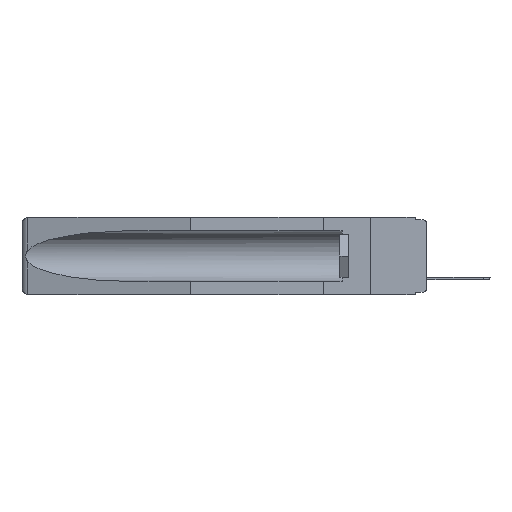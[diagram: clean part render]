
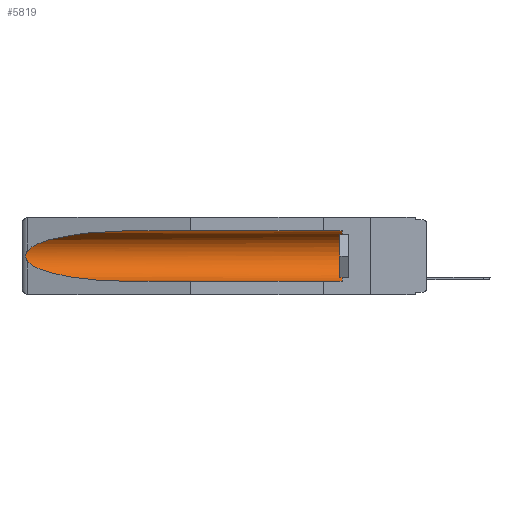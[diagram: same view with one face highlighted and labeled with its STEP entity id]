
A CAD part, left-side view. The second image highlights one B-rep face of the part: STEP entity #5819.
In plain terms, the highlighted cylindrical face has radius 2.857 mm (diameter 5.715 mm), a partial arc.
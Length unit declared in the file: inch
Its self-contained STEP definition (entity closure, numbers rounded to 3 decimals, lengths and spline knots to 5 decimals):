
#19 = CARTESIAN_POINT ( 'NONE',  ( 0.26537, 1.52718, -0.19328 ) ) ;
#330 = CARTESIAN_POINT ( 'NONE',  ( 0.26537, 1.52718, -0.14972 ) ) ;
#913 = EDGE_CURVE ( 'NONE', #8748, #20249, #10595, .T. ) ;
#1345 = DIRECTION ( 'NONE',  ( 0., -1., 0. ) ) ;
#2496 = B_SPLINE_CURVE_WITH_KNOTS ( 'NONE', 3,
 ( #20690, #14370, #4111, #4431, #2580, #7816, #5740, #9347, #16097, #19382 ),
 .UNSPECIFIED., .F., .F.,
 ( 4, 2, 2, 2, 4 ),
 ( 0., 0.00029, 0.00058, 0.00087, 0.00117 ),
 .UNSPECIFIED. ) ;
#2580 = CARTESIAN_POINT ( 'NONE',  ( 0.2675, 1.53308, -0.16763 ) ) ;
#3056 = EDGE_CURVE ( 'NONE', #6272, #9752, #18085, .T. ) ;
#3362 = CARTESIAN_POINT ( 'NONE',  ( 0.155, 0.126, -0.284 ) ) ;
#3467 = CARTESIAN_POINT ( 'NONE',  ( 0.26537, 1.52718, -0.14972 ) ) ;
#4111 = CARTESIAN_POINT ( 'NONE',  ( 0.26654, 1.53092, -0.15636 ) ) ;
#4431 = CARTESIAN_POINT ( 'NONE',  ( 0.2673, 1.5327, -0.16383 ) ) ;
#4474 = LINE ( 'NONE', #6005, #21567 ) ;
#4707 = CARTESIAN_POINT ( 'NONE',  ( 0.155, -0.30754, -0.284 ) ) ;
#4828 = ORIENTED_EDGE ( 'NONE', *, *, #12838, .T. ) ;
#4932 = CIRCLE ( 'NONE', #10875, 0.1125 ) ;
#5128 = CARTESIAN_POINT ( 'NONE',  ( 0.155, 0.126, -0.1715 ) ) ;
#5740 = CARTESIAN_POINT ( 'NONE',  ( 0.2673, 1.53269, -0.17917 ) ) ;
#5819 = ADVANCED_FACE ( 'NONE', ( #16877 ), #18187, .F. ) ;
#6005 = CARTESIAN_POINT ( 'NONE',  ( 0.155, -0.30754, -0.059 ) ) ;
#6249 = CARTESIAN_POINT ( 'NONE',  ( 0.155, 1.07973, -0.284 ) ) ;
#6272 = VERTEX_POINT ( 'NONE', #6819 ) ;
#6819 = CARTESIAN_POINT ( 'NONE',  ( 0.155, 1.07973, -0.059 ) ) ;
#7217 = VERTEX_POINT ( 'NONE', #3362 ) ;
#7816 = CARTESIAN_POINT ( 'NONE',  ( 0.2675, 1.53308, -0.17534 ) ) ;
#8462 = EDGE_CURVE ( 'NONE', #7217, #20249, #18228, .T. ) ;
#8748 = VERTEX_POINT ( 'NONE', #14078 ) ;
#9347 = CARTESIAN_POINT ( 'NONE',  ( 0.26655, 1.53094, -0.18657 ) ) ;
#9752 = VERTEX_POINT ( 'NONE', #330 ) ;
#10130 = CARTESIAN_POINT ( 'NONE',  ( 0.21114, 1.30732, -0.059 ) ) ;
#10202 = AXIS2_PLACEMENT_3D ( 'NONE', #20037, #19814, #16764 ) ;
#10595 =( BOUNDED_CURVE ( )  B_SPLINE_CURVE ( 3, ( #19, #13235, #15093, #18135 ),
 .UNSPECIFIED., .F., .F. ) 
 B_SPLINE_CURVE_WITH_KNOTS ( ( 4, 4 ),
 ( 0.1948, 1.5708 ),
 .UNSPECIFIED. ) 
 CURVE ( )  GEOMETRIC_REPRESENTATION_ITEM ( )  RATIONAL_B_SPLINE_CURVE ( ( 1., 0.848, 0.848, 1. ) ) 
 REPRESENTATION_ITEM ( '' )  );
#10875 = AXIS2_PLACEMENT_3D ( 'NONE', #5128, #1345, #14562 ) ;
#11068 = ORIENTED_EDGE ( 'NONE', *, *, #913, .T. ) ;
#11891 = CARTESIAN_POINT ( 'NONE',  ( 0.155, 1.07973, -0.059 ) ) ;
#12295 = EDGE_LOOP ( 'NONE', ( #13754, #18700, #11068, #17806, #17224, #4828 ) ) ;
#12838 = EDGE_CURVE ( 'NONE', #15915, #6272, #4474, .T. ) ;
#13235 = CARTESIAN_POINT ( 'NONE',  ( 0.25451, 1.48313, -0.24835 ) ) ;
#13754 = ORIENTED_EDGE ( 'NONE', *, *, #3056, .T. ) ;
#14078 = CARTESIAN_POINT ( 'NONE',  ( 0.26537, 1.52718, -0.19328 ) ) ;
#14309 = DIRECTION ( 'NONE',  ( 0., 1., 0. ) ) ;
#14370 = CARTESIAN_POINT ( 'NONE',  ( 0.26597, 1.52961, -0.15275 ) ) ;
#14562 = DIRECTION ( 'NONE',  ( 0., 0., 1. ) ) ;
#14902 = EDGE_CURVE ( 'NONE', #9752, #8748, #2496, .T. ) ;
#14932 = CARTESIAN_POINT ( 'NONE',  ( 0.25451, 1.48313, -0.09465 ) ) ;
#15093 = CARTESIAN_POINT ( 'NONE',  ( 0.21114, 1.30732, -0.284 ) ) ;
#15915 = VERTEX_POINT ( 'NONE', #18199 ) ;
#16097 = CARTESIAN_POINT ( 'NONE',  ( 0.26597, 1.5296, -0.19026 ) ) ;
#16764 = DIRECTION ( 'NONE',  ( 0., 0., 1. ) ) ;
#16877 = FACE_OUTER_BOUND ( 'NONE', #12295, .T. ) ;
#17224 = ORIENTED_EDGE ( 'NONE', *, *, #20211, .T. ) ;
#17806 = ORIENTED_EDGE ( 'NONE', *, *, #8462, .F. ) ;
#18085 =( BOUNDED_CURVE ( )  B_SPLINE_CURVE ( 3, ( #11891, #10130, #14932, #3467 ),
 .UNSPECIFIED., .F., .T. ) 
 B_SPLINE_CURVE_WITH_KNOTS ( ( 4, 4 ),
 ( 4.71239, 6.08839 ),
 .UNSPECIFIED. ) 
 CURVE ( )  GEOMETRIC_REPRESENTATION_ITEM ( )  RATIONAL_B_SPLINE_CURVE ( ( 1., 0.848, 0.848, 1. ) ) 
 REPRESENTATION_ITEM ( '' )  );
#18135 = CARTESIAN_POINT ( 'NONE',  ( 0.155, 1.07973, -0.284 ) ) ;
#18187 = CYLINDRICAL_SURFACE ( 'NONE', #10202, 0.1125 ) ;
#18199 = CARTESIAN_POINT ( 'NONE',  ( 0.155, 0.126, -0.059 ) ) ;
#18228 = LINE ( 'NONE', #4707, #20047 ) ;
#18700 = ORIENTED_EDGE ( 'NONE', *, *, #14902, .T. ) ;
#19382 = CARTESIAN_POINT ( 'NONE',  ( 0.26537, 1.52718, -0.19328 ) ) ;
#19540 = DIRECTION ( 'NONE',  ( 0., 1., 0. ) ) ;
#19814 = DIRECTION ( 'NONE',  ( 0., 1., 0. ) ) ;
#20037 = CARTESIAN_POINT ( 'NONE',  ( 0.155, -0.30754, -0.1715 ) ) ;
#20047 = VECTOR ( 'NONE', #19540, 39.37008 ) ;
#20211 = EDGE_CURVE ( 'NONE', #7217, #15915, #4932, .T. ) ;
#20249 = VERTEX_POINT ( 'NONE', #6249 ) ;
#20690 = CARTESIAN_POINT ( 'NONE',  ( 0.26537, 1.52718, -0.14972 ) ) ;
#21567 = VECTOR ( 'NONE', #14309, 39.37008 ) ;
